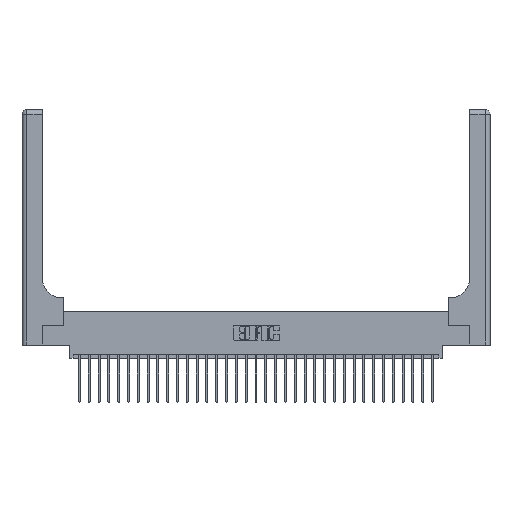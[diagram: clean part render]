
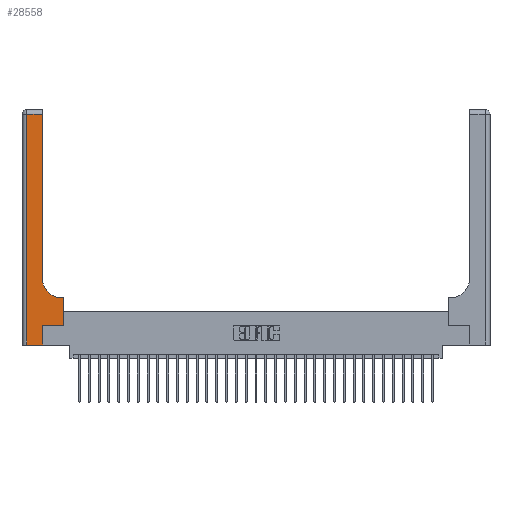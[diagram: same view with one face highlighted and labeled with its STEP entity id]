
A CAD part, top view. The second image highlights one B-rep face of the part: STEP entity #28558.
In plain terms, the highlighted planar face has unit normal (0, 0, 1).
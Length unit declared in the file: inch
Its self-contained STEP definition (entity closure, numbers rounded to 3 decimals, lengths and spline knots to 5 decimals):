
#799 = EDGE_CURVE ( 'NONE', #4197, #5139, #832, .T. ) ;
#832 = LINE ( 'NONE', #21527, #18711 ) ;
#1127 = LINE ( 'NONE', #2445, #19015 ) ;
#1201 = CARTESIAN_POINT ( 'NONE',  ( 0.265, 0.25, 0.37 ) ) ;
#1475 = LINE ( 'NONE', #28640, #25581 ) ;
#2025 = VECTOR ( 'NONE', #18110, 39.37008 ) ;
#2248 = CARTESIAN_POINT ( 'NONE',  ( 0.06, 2.94, 0.37 ) ) ;
#2445 = CARTESIAN_POINT ( 'NONE',  ( 0.265, 0., 0.37 ) ) ;
#2790 = LINE ( 'NONE', #6510, #3506 ) ;
#3351 = EDGE_LOOP ( 'NONE', ( #3988, #3511, #28220, #23653, #10848, #23499, #5612, #4669, #13902 ) ) ;
#3506 = VECTOR ( 'NONE', #25088, 39.37008 ) ;
#3511 = ORIENTED_EDGE ( 'NONE', *, *, #16436, .T. ) ;
#3546 = DIRECTION ( 'NONE',  ( 1., 0., 0. ) ) ;
#3579 = DIRECTION ( 'NONE',  ( -1., 0., 0. ) ) ;
#3988 = ORIENTED_EDGE ( 'NONE', *, *, #9245, .T. ) ;
#4079 = CARTESIAN_POINT ( 'NONE',  ( 0.265, 0., 0.37 ) ) ;
#4197 = VERTEX_POINT ( 'NONE', #2248 ) ;
#4669 = ORIENTED_EDGE ( 'NONE', *, *, #20681, .T. ) ;
#5139 = VERTEX_POINT ( 'NONE', #17782 ) ;
#5612 = ORIENTED_EDGE ( 'NONE', *, *, #11006, .T. ) ;
#6297 = CARTESIAN_POINT ( 'NONE',  ( 0.51, 0.6, 0.37 ) ) ;
#6510 = CARTESIAN_POINT ( 'NONE',  ( 0., 2.94, 0.37 ) ) ;
#8003 = CARTESIAN_POINT ( 'NONE',  ( 0.51, 0.85, 0.37 ) ) ;
#8296 = CARTESIAN_POINT ( 'NONE',  ( 0., 0., 0.37 ) ) ;
#8939 = LINE ( 'NONE', #8296, #2025 ) ;
#9194 = EDGE_CURVE ( 'NONE', #20825, #21541, #11805, .T. ) ;
#9245 = EDGE_CURVE ( 'NONE', #21541, #10631, #28239, .T. ) ;
#9664 = VERTEX_POINT ( 'NONE', #21781 ) ;
#10357 = DIRECTION ( 'NONE',  ( 1., 0., 0. ) ) ;
#10631 = VERTEX_POINT ( 'NONE', #24989 ) ;
#10821 = EDGE_CURVE ( 'NONE', #29634, #27158, #1127, .T. ) ;
#10848 = ORIENTED_EDGE ( 'NONE', *, *, #10821, .T. ) ;
#11006 = EDGE_CURVE ( 'NONE', #13169, #9664, #1475, .T. ) ;
#11805 = CIRCLE ( 'NONE', #12699, 0.25 ) ;
#12409 = DIRECTION ( 'NONE',  ( 0., 1., 0. ) ) ;
#12521 = CARTESIAN_POINT ( 'NONE',  ( 0.26, 0.6, 0.37 ) ) ;
#12699 = AXIS2_PLACEMENT_3D ( 'NONE', #8003, #24344, #10357 ) ;
#12769 = FACE_OUTER_BOUND ( 'NONE', #3351, .T. ) ;
#12872 = PLANE ( 'NONE',  #18139 ) ;
#13169 = VERTEX_POINT ( 'NONE', #19084 ) ;
#13902 = ORIENTED_EDGE ( 'NONE', *, *, #9194, .T. ) ;
#14868 = DIRECTION ( 'NONE',  ( -1., 0., 0. ) ) ;
#15222 = CARTESIAN_POINT ( 'NONE',  ( 0., 3., 0.37 ) ) ;
#16409 = DIRECTION ( 'NONE',  ( 0., 1., 0. ) ) ;
#16436 = EDGE_CURVE ( 'NONE', #10631, #4197, #2790, .T. ) ;
#16571 = CARTESIAN_POINT ( 'NONE',  ( 0.26, 0.85, 0.37 ) ) ;
#16824 = CARTESIAN_POINT ( 'NONE',  ( 0.265, 0.25, 0.37 ) ) ;
#16916 = EDGE_CURVE ( 'NONE', #5139, #29634, #8939, .T. ) ;
#17115 = VECTOR ( 'NONE', #3546, 39.37008 ) ;
#17496 = DIRECTION ( 'NONE',  ( 0., 1., 0. ) ) ;
#17569 = DIRECTION ( 'NONE',  ( 0., 0., -1. ) ) ;
#17782 = CARTESIAN_POINT ( 'NONE',  ( 0.06, 0., 0.37 ) ) ;
#18110 = DIRECTION ( 'NONE',  ( 1., 0., 0. ) ) ;
#18139 = AXIS2_PLACEMENT_3D ( 'NONE', #15222, #17569, #3579 ) ;
#18711 = VECTOR ( 'NONE', #23868, 39.37008 ) ;
#19015 = VECTOR ( 'NONE', #16409, 39.37008 ) ;
#19084 = CARTESIAN_POINT ( 'NONE',  ( 0.528, 0.25, 0.37 ) ) ;
#20681 = EDGE_CURVE ( 'NONE', #9664, #20825, #28975, .T. ) ;
#20825 = VERTEX_POINT ( 'NONE', #6297 ) ;
#21527 = CARTESIAN_POINT ( 'NONE',  ( 0.06, 3., 0.37 ) ) ;
#21541 = VERTEX_POINT ( 'NONE', #16571 ) ;
#21781 = CARTESIAN_POINT ( 'NONE',  ( 0.528, 0.6, 0.37 ) ) ;
#22051 = VECTOR ( 'NONE', #17496, 39.37008 ) ;
#22076 = VECTOR ( 'NONE', #14868, 39.37008 ) ;
#23332 = LINE ( 'NONE', #1201, #17115 ) ;
#23499 = ORIENTED_EDGE ( 'NONE', *, *, #30053, .T. ) ;
#23653 = ORIENTED_EDGE ( 'NONE', *, *, #16916, .T. ) ;
#23868 = DIRECTION ( 'NONE',  ( 0., -1., 0. ) ) ;
#24344 = DIRECTION ( 'NONE',  ( 0., 0., -1. ) ) ;
#24445 = CARTESIAN_POINT ( 'NONE',  ( 0.26, 3., 0.37 ) ) ;
#24989 = CARTESIAN_POINT ( 'NONE',  ( 0.26, 2.94, 0.37 ) ) ;
#25088 = DIRECTION ( 'NONE',  ( -1., 0., 0. ) ) ;
#25581 = VECTOR ( 'NONE', #12409, 39.37008 ) ;
#27158 = VERTEX_POINT ( 'NONE', #16824 ) ;
#28220 = ORIENTED_EDGE ( 'NONE', *, *, #799, .T. ) ;
#28239 = LINE ( 'NONE', #24445, #22051 ) ;
#28558 = ADVANCED_FACE ( 'NONE', ( #12769 ), #12872, .F. ) ;
#28640 = CARTESIAN_POINT ( 'NONE',  ( 0.528, 0.25, 0.37 ) ) ;
#28975 = LINE ( 'NONE', #12521, #22076 ) ;
#29634 = VERTEX_POINT ( 'NONE', #4079 ) ;
#30053 = EDGE_CURVE ( 'NONE', #27158, #13169, #23332, .T. ) ;
